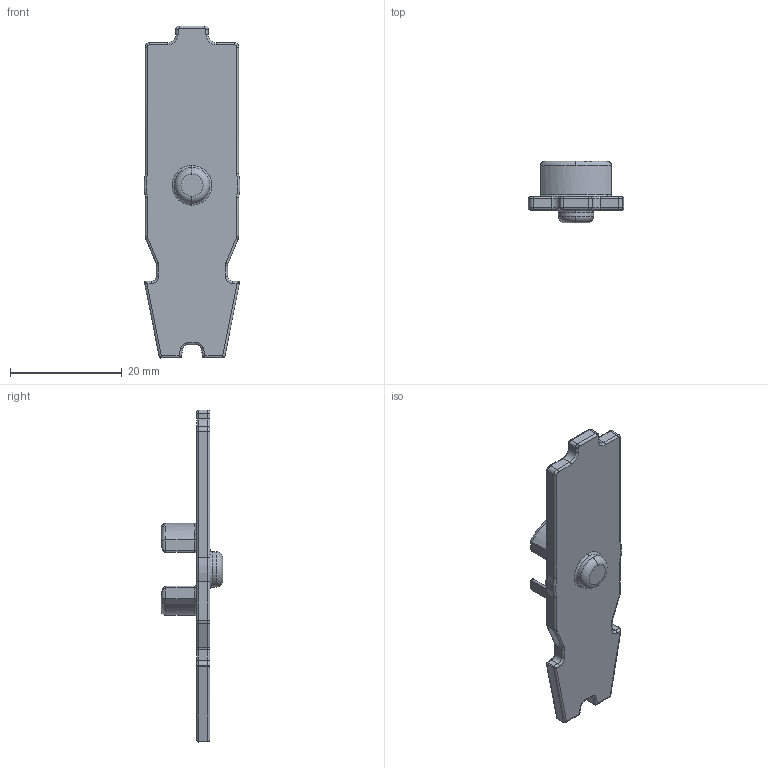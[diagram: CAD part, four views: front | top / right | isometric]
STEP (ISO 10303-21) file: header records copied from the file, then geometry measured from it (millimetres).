
FILE_DESCRIPTION(/* description */ ('STEP AP214'),/* implementation_level */ '2;1');
FILE_NAME(/* name */ 'Ivan''Ivan''s Standard Mag Locking Plate.stp',/* time_stamp */ '2019-01-27T20:55:08-06:00',/* author */ ('johne'),/* organization */ (''),/* preprocessor_version */ 'ST-DEVELOPER v16.13',/* originating_system */ 'Autodesk Inventor 2018',/* authorisation */ '');
FILE_SCHEMA (('AUTOMOTIVE_DESIGN { 1 0 10303 214 3 1 1 }'));
Length unit declared in the file: inch
Products named in the file (1): DefDist_Cuomo_AR15_30_Mag_Spring_Base
Bounding box: 17.21 x 11.02 x 59.54 mm (x, y, z)
Volume: 2508.9 mm3; surface area: 2550.8 mm2
Topology: 1 solids, 1 shells, 182 faces, 421 edges, 228 vertices
Faces by surface type: cylinder 83, torus 50, plane 29, bspline 20
Full cylindrical faces by diameter (mm): 6.35 x1
Entity records: 7088 total; most frequent: CARTESIAN_POINT 3111, DIRECTION 864, ORIENTED_EDGE 808, EDGE_CURVE 404, AXIS2_PLACEMENT_3D 354, VERTEX_POINT 228, CIRCLE 188, EDGE_LOOP 186
